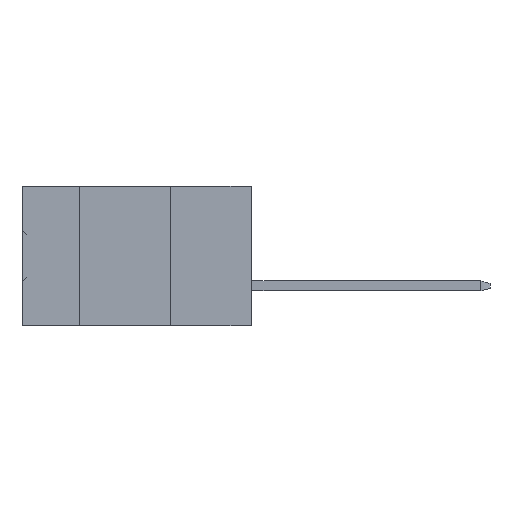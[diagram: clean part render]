
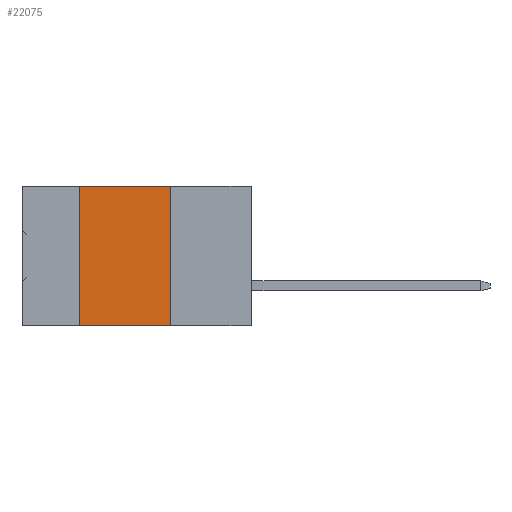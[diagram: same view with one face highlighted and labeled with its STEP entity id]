
A CAD part, left-side view. The second image highlights one B-rep face of the part: STEP entity #22075.
In plain terms, the highlighted planar face has unit normal (-1, 0, 0).
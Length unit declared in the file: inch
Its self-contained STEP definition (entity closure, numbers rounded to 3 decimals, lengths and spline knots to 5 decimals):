
#665 = AXIS2_PLACEMENT_3D ( 'NONE', #4074, #23294, #11291 ) ;
#1057 = EDGE_CURVE ( 'NONE', #13741, #6833, #18117, .T. ) ;
#1212 = LINE ( 'NONE', #7940, #25549 ) ;
#3765 = DIRECTION ( 'NONE',  ( 0., -1., 0. ) ) ;
#4074 = CARTESIAN_POINT ( 'NONE',  ( 0., 0.72, 0. ) ) ;
#4378 = ORIENTED_EDGE ( 'NONE', *, *, #20874, .F. ) ;
#6046 = VECTOR ( 'NONE', #28308, 39.37008 ) ;
#6806 = EDGE_LOOP ( 'NONE', ( #12943, #29592, #4378, #18757 ) ) ;
#6833 = VERTEX_POINT ( 'NONE', #24189 ) ;
#7940 = CARTESIAN_POINT ( 'NONE',  ( 0., 0.254, -0.437 ) ) ;
#9666 = LINE ( 'NONE', #11588, #6046 ) ;
#11291 = DIRECTION ( 'NONE',  ( 0., 0., -1. ) ) ;
#11588 = CARTESIAN_POINT ( 'NONE',  ( 0., 0.72, 0. ) ) ;
#12943 = ORIENTED_EDGE ( 'NONE', *, *, #28255, .F. ) ;
#13741 = VERTEX_POINT ( 'NONE', #30059 ) ;
#16055 = PLANE ( 'NONE',  #665 ) ;
#16672 = DIRECTION ( 'NONE',  ( 0., 0., 1. ) ) ;
#18117 = LINE ( 'NONE', #22673, #25280 ) ;
#18757 = ORIENTED_EDGE ( 'NONE', *, *, #1057, .T. ) ;
#18872 = LINE ( 'NONE', #28622, #25220 ) ;
#18906 = EDGE_CURVE ( 'NONE', #22480, #20352, #9666, .T. ) ;
#20352 = VERTEX_POINT ( 'NONE', #27741 ) ;
#20874 = EDGE_CURVE ( 'NONE', #13741, #22480, #18872, .T. ) ;
#22075 = ADVANCED_FACE ( 'NONE', ( #25471 ), #16055, .F. ) ;
#22480 = VERTEX_POINT ( 'NONE', #25274 ) ;
#22612 = DIRECTION ( 'NONE',  ( 0., 0., -1. ) ) ;
#22673 = CARTESIAN_POINT ( 'NONE',  ( 0., 0.72, -0.437 ) ) ;
#23294 = DIRECTION ( 'NONE',  ( 1., 0., 0. ) ) ;
#24189 = CARTESIAN_POINT ( 'NONE',  ( 0., 0.254, -0.437 ) ) ;
#25220 = VECTOR ( 'NONE', #16672, 39.37008 ) ;
#25274 = CARTESIAN_POINT ( 'NONE',  ( 0., 0.54, 0. ) ) ;
#25280 = VECTOR ( 'NONE', #3765, 39.37008 ) ;
#25471 = FACE_OUTER_BOUND ( 'NONE', #6806, .T. ) ;
#25549 = VECTOR ( 'NONE', #22612, 39.37008 ) ;
#27741 = CARTESIAN_POINT ( 'NONE',  ( 0., 0.254, 0. ) ) ;
#28255 = EDGE_CURVE ( 'NONE', #20352, #6833, #1212, .T. ) ;
#28308 = DIRECTION ( 'NONE',  ( 0., -1., 0. ) ) ;
#28622 = CARTESIAN_POINT ( 'NONE',  ( 0., 0.54, -0.437 ) ) ;
#29592 = ORIENTED_EDGE ( 'NONE', *, *, #18906, .F. ) ;
#30059 = CARTESIAN_POINT ( 'NONE',  ( 0., 0.54, -0.437 ) ) ;
